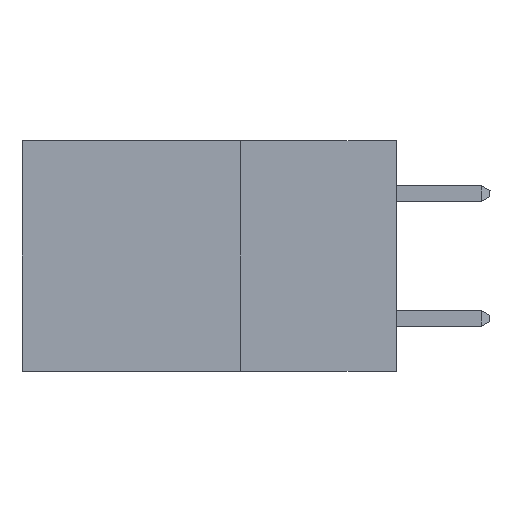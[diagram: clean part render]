
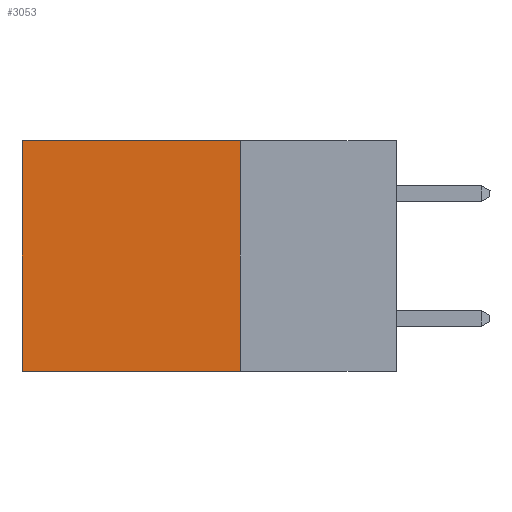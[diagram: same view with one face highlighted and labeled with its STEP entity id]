
A CAD part, left-side view. The second image highlights one B-rep face of the part: STEP entity #3053.
In plain terms, the highlighted planar face has unit normal (-1, 0, 0).
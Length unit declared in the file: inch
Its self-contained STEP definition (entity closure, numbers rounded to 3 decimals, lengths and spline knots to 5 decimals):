
#14 = VERTEX_POINT ( 'NONE', #3782 ) ;
#478 = CARTESIAN_POINT ( 'NONE',  ( 0.298, 0.25, -0.37 ) ) ;
#796 = CARTESIAN_POINT ( 'NONE',  ( 0.298, 0.25, 0. ) ) ;
#843 = LINE ( 'NONE', #6548, #2838 ) ;
#996 = ORIENTED_EDGE ( 'NONE', *, *, #2783, .T. ) ;
#1066 = EDGE_CURVE ( 'NONE', #10267, #1428, #7794, .T. ) ;
#1256 = CARTESIAN_POINT ( 'NONE',  ( 0.298, 0.25, -0.37 ) ) ;
#1399 = VERTEX_POINT ( 'NONE', #796 ) ;
#1428 = VERTEX_POINT ( 'NONE', #4060 ) ;
#2783 = EDGE_CURVE ( 'NONE', #1399, #14, #843, .T. ) ;
#2838 = VECTOR ( 'NONE', #6806, 39.37008 ) ;
#3053 = ADVANCED_FACE ( 'NONE', ( #5132 ), #6522, .F. ) ;
#3085 = VECTOR ( 'NONE', #8595, 39.37008 ) ;
#3206 = EDGE_CURVE ( 'NONE', #1399, #10267, #9476, .T. ) ;
#3782 = CARTESIAN_POINT ( 'NONE',  ( 0.298, 0.6, 0. ) ) ;
#4060 = CARTESIAN_POINT ( 'NONE',  ( 0.298, 0.6, -0.37 ) ) ;
#4856 = DIRECTION ( 'NONE',  ( 0., 0., -1. ) ) ;
#5132 = FACE_OUTER_BOUND ( 'NONE', #10530, .T. ) ;
#5670 = VECTOR ( 'NONE', #8810, 39.37008 ) ;
#5945 = LINE ( 'NONE', #8013, #7827 ) ;
#6273 = CARTESIAN_POINT ( 'NONE',  ( 0.298, 0.25, 0. ) ) ;
#6365 = DIRECTION ( 'NONE',  ( 0., 0., -1. ) ) ;
#6379 = DIRECTION ( 'NONE',  ( 1., 0., 0. ) ) ;
#6522 = PLANE ( 'NONE',  #9846 ) ;
#6548 = CARTESIAN_POINT ( 'NONE',  ( 0.298, 0.25, 0. ) ) ;
#6806 = DIRECTION ( 'NONE',  ( 0., 1., 0. ) ) ;
#7104 = ORIENTED_EDGE ( 'NONE', *, *, #1066, .F. ) ;
#7734 = ORIENTED_EDGE ( 'NONE', *, *, #8071, .T. ) ;
#7794 = LINE ( 'NONE', #478, #5670 ) ;
#7827 = VECTOR ( 'NONE', #4856, 39.37008 ) ;
#7851 = ORIENTED_EDGE ( 'NONE', *, *, #3206, .F. ) ;
#8013 = CARTESIAN_POINT ( 'NONE',  ( 0.298, 0.6, 0. ) ) ;
#8071 = EDGE_CURVE ( 'NONE', #14, #1428, #5945, .T. ) ;
#8395 = CARTESIAN_POINT ( 'NONE',  ( 0.298, 0.25, 0. ) ) ;
#8595 = DIRECTION ( 'NONE',  ( 0., 0., -1. ) ) ;
#8810 = DIRECTION ( 'NONE',  ( 0., 1., 0. ) ) ;
#9476 = LINE ( 'NONE', #8395, #3085 ) ;
#9846 = AXIS2_PLACEMENT_3D ( 'NONE', #6273, #6379, #6365 ) ;
#10267 = VERTEX_POINT ( 'NONE', #1256 ) ;
#10530 = EDGE_LOOP ( 'NONE', ( #7734, #7104, #7851, #996 ) ) ;
